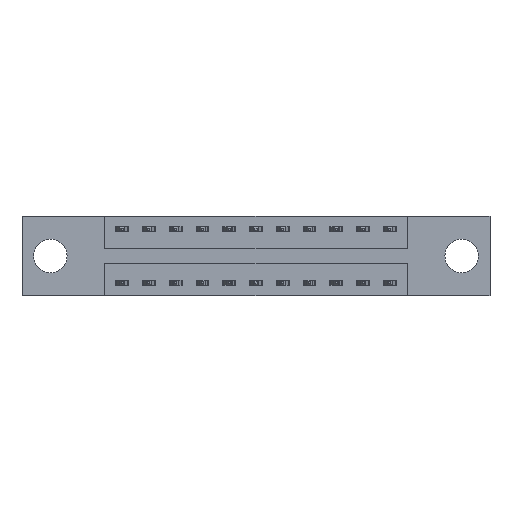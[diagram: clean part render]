
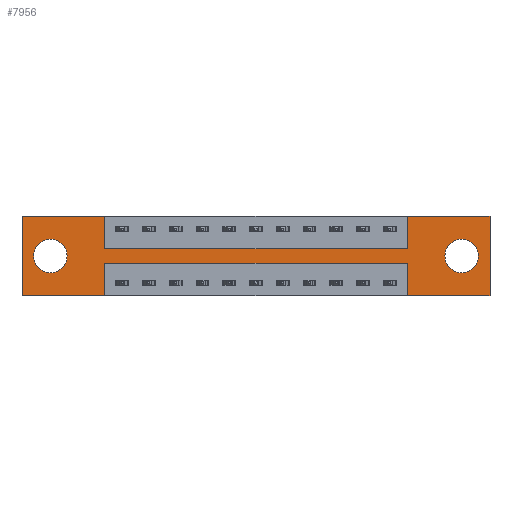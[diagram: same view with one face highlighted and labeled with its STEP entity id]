
A CAD part, front view. The second image highlights one B-rep face of the part: STEP entity #7956.
In plain terms, the highlighted planar face has unit normal (0, -1, 0).
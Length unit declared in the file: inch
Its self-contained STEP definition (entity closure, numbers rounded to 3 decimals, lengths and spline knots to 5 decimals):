
#3 = VERTEX_POINT ( 'NONE', #10753 ) ;
#63 = CARTESIAN_POINT ( 'NONE',  ( 0., 0., 0. ) ) ;
#171 = VECTOR ( 'NONE', #5956, 39.37008 ) ;
#197 = AXIS2_PLACEMENT_3D ( 'NONE', #10692, #4451, #8033 ) ;
#284 = CARTESIAN_POINT ( 'NONE',  ( 0.3875, 0., -0.22 ) ) ;
#301 = VERTEX_POINT ( 'NONE', #1676 ) ;
#316 = LINE ( 'NONE', #10496, #5406 ) ;
#406 = DIRECTION ( 'NONE',  ( 0., 1., 0. ) ) ;
#453 = ORIENTED_EDGE ( 'NONE', *, *, #6720, .F. ) ;
#528 = LINE ( 'NONE', #2189, #7311 ) ;
#599 = EDGE_CURVE ( 'NONE', #2090, #2115, #6067, .T. ) ;
#660 = PLANE ( 'NONE',  #197 ) ;
#682 = EDGE_CURVE ( 'NONE', #7720, #2903, #2788, .T. ) ;
#719 = EDGE_CURVE ( 'NONE', #2115, #2090, #3470, .T. ) ;
#831 = ORIENTED_EDGE ( 'NONE', *, *, #599, .T. ) ;
#849 = DIRECTION ( 'NONE',  ( 1., 0., 0. ) ) ;
#893 = DIRECTION ( 'NONE',  ( 0., 0., 1. ) ) ;
#897 = CARTESIAN_POINT ( 'NONE',  ( 0., 0., 0. ) ) ;
#911 = DIRECTION ( 'NONE',  ( 0., 0., 1. ) ) ;
#1139 = VECTOR ( 'NONE', #849, 39.37008 ) ;
#1198 = EDGE_CURVE ( 'NONE', #301, #8173, #5042, .T. ) ;
#1199 = DIRECTION ( 'NONE',  ( 0., 0., -1. ) ) ;
#1268 = DIRECTION ( 'NONE',  ( 0., 0., 1. ) ) ;
#1390 = DIRECTION ( 'NONE',  ( 0., 0., 1. ) ) ;
#1467 = VERTEX_POINT ( 'NONE', #3126 ) ;
#1552 = EDGE_CURVE ( 'NONE', #8173, #11756, #1583, .T. ) ;
#1583 = LINE ( 'NONE', #8945, #7128 ) ;
#1618 = ORIENTED_EDGE ( 'NONE', *, *, #719, .T. ) ;
#1676 = CARTESIAN_POINT ( 'NONE',  ( 1.7975, 0., -0.22 ) ) ;
#1816 = CARTESIAN_POINT ( 'NONE',  ( 2.0525, 0., -0.185 ) ) ;
#1943 = EDGE_CURVE ( 'NONE', #8447, #10430, #528, .T. ) ;
#2009 = EDGE_LOOP ( 'NONE', ( #1618, #831 ) ) ;
#2090 = VERTEX_POINT ( 'NONE', #11554 ) ;
#2115 = VERTEX_POINT ( 'NONE', #11005 ) ;
#2189 = CARTESIAN_POINT ( 'NONE',  ( 1.7975, 0., 0. ) ) ;
#2198 = ORIENTED_EDGE ( 'NONE', *, *, #1943, .F. ) ;
#2272 = AXIS2_PLACEMENT_3D ( 'NONE', #1816, #10988, #4686 ) ;
#2542 = VECTOR ( 'NONE', #7176, 39.37008 ) ;
#2788 = CIRCLE ( 'NONE', #10958, 0.078 ) ;
#2804 = CARTESIAN_POINT ( 'NONE',  ( 0., 0., -0.37 ) ) ;
#2903 = VERTEX_POINT ( 'NONE', #10499 ) ;
#2908 = VERTEX_POINT ( 'NONE', #7887 ) ;
#2961 = VECTOR ( 'NONE', #8928, 39.37008 ) ;
#3126 = CARTESIAN_POINT ( 'NONE',  ( 1.7975, 0., -0.37 ) ) ;
#3278 = ORIENTED_EDGE ( 'NONE', *, *, #5797, .T. ) ;
#3384 = LINE ( 'NONE', #7021, #11102 ) ;
#3470 = CIRCLE ( 'NONE', #2272, 0.078 ) ;
#3542 = LINE ( 'NONE', #4397, #2542 ) ;
#3602 = LINE ( 'NONE', #897, #11501 ) ;
#3729 = LINE ( 'NONE', #2804, #4308 ) ;
#3768 = VECTOR ( 'NONE', #911, 39.37008 ) ;
#3975 = AXIS2_PLACEMENT_3D ( 'NONE', #11304, #406, #1199 ) ;
#4032 = DIRECTION ( 'NONE',  ( -1., 0., 0. ) ) ;
#4108 = ORIENTED_EDGE ( 'NONE', *, *, #1198, .F. ) ;
#4280 = VERTEX_POINT ( 'NONE', #6567 ) ;
#4308 = VECTOR ( 'NONE', #4515, 39.37008 ) ;
#4397 = CARTESIAN_POINT ( 'NONE',  ( 0.3875, 0., -0.15 ) ) ;
#4451 = DIRECTION ( 'NONE',  ( 0., -1., 0. ) ) ;
#4515 = DIRECTION ( 'NONE',  ( -1., 0., 0. ) ) ;
#4624 = ORIENTED_EDGE ( 'NONE', *, *, #4919, .F. ) ;
#4686 = DIRECTION ( 'NONE',  ( 0., 0., -1. ) ) ;
#4919 = EDGE_CURVE ( 'NONE', #11756, #6118, #3729, .T. ) ;
#4962 = ORIENTED_EDGE ( 'NONE', *, *, #682, .T. ) ;
#5030 = AXIS2_PLACEMENT_3D ( 'NONE', #5996, #9581, #1390 ) ;
#5042 = LINE ( 'NONE', #284, #7092 ) ;
#5107 = EDGE_CURVE ( 'NONE', #2908, #1467, #316, .T. ) ;
#5137 = VERTEX_POINT ( 'NONE', #5603 ) ;
#5223 = CIRCLE ( 'NONE', #5030, 0.078 ) ;
#5257 = CARTESIAN_POINT ( 'NONE',  ( 0.3875, 0., -0.15 ) ) ;
#5369 = CARTESIAN_POINT ( 'NONE',  ( 0.1325, 0., -0.107 ) ) ;
#5406 = VECTOR ( 'NONE', #5784, 39.37008 ) ;
#5572 = DIRECTION ( 'NONE',  ( 0., 1., 0. ) ) ;
#5603 = CARTESIAN_POINT ( 'NONE',  ( 0., 0., 0. ) ) ;
#5784 = DIRECTION ( 'NONE',  ( -1., 0., 0. ) ) ;
#5797 = EDGE_CURVE ( 'NONE', #2903, #7720, #5223, .T. ) ;
#5956 = DIRECTION ( 'NONE',  ( 0., 0., -1. ) ) ;
#5996 = CARTESIAN_POINT ( 'NONE',  ( 0.1325, 0., -0.185 ) ) ;
#6010 = CARTESIAN_POINT ( 'NONE',  ( 0.3875, 0., -0.37 ) ) ;
#6067 = CIRCLE ( 'NONE', #3975, 0.078 ) ;
#6118 = VERTEX_POINT ( 'NONE', #7252 ) ;
#6434 = ORIENTED_EDGE ( 'NONE', *, *, #8017, .F. ) ;
#6445 = ORIENTED_EDGE ( 'NONE', *, *, #1552, .F. ) ;
#6567 = CARTESIAN_POINT ( 'NONE',  ( 0.3875, 0., 0. ) ) ;
#6720 = EDGE_CURVE ( 'NONE', #4280, #11645, #8645, .T. ) ;
#6988 = CARTESIAN_POINT ( 'NONE',  ( 0.1325, 0., -0.185 ) ) ;
#7021 = CARTESIAN_POINT ( 'NONE',  ( 1.7975, 0., -0.37 ) ) ;
#7092 = VECTOR ( 'NONE', #4032, 39.37008 ) ;
#7108 = DIRECTION ( 'NONE',  ( 0., 0., -1. ) ) ;
#7128 = VECTOR ( 'NONE', #7108, 39.37008 ) ;
#7176 = DIRECTION ( 'NONE',  ( 1., 0., 0. ) ) ;
#7252 = CARTESIAN_POINT ( 'NONE',  ( 0., 0., -0.37 ) ) ;
#7311 = VECTOR ( 'NONE', #1268, 39.37008 ) ;
#7344 = LINE ( 'NONE', #63, #1139 ) ;
#7414 = CARTESIAN_POINT ( 'NONE',  ( 1.7975, 0., 0. ) ) ;
#7705 = ORIENTED_EDGE ( 'NONE', *, *, #11022, .F. ) ;
#7720 = VERTEX_POINT ( 'NONE', #5369 ) ;
#7844 = CARTESIAN_POINT ( 'NONE',  ( 1.7975, 0., -0.15 ) ) ;
#7887 = CARTESIAN_POINT ( 'NONE',  ( 2.185, 0., -0.37 ) ) ;
#7956 = ADVANCED_FACE ( 'NONE', ( #11494, #9810, #8873 ), #660, .T. ) ;
#8017 = EDGE_CURVE ( 'NONE', #5137, #4280, #7344, .T. ) ;
#8030 = ORIENTED_EDGE ( 'NONE', *, *, #10691, .F. ) ;
#8033 = DIRECTION ( 'NONE',  ( 0., 0., -1. ) ) ;
#8098 = ORIENTED_EDGE ( 'NONE', *, *, #9677, .F. ) ;
#8167 = CARTESIAN_POINT ( 'NONE',  ( 0., 0., 0. ) ) ;
#8173 = VERTEX_POINT ( 'NONE', #9857 ) ;
#8220 = ORIENTED_EDGE ( 'NONE', *, *, #5107, .F. ) ;
#8447 = VERTEX_POINT ( 'NONE', #7844 ) ;
#8493 = ORIENTED_EDGE ( 'NONE', *, *, #10370, .F. ) ;
#8516 = EDGE_LOOP ( 'NONE', ( #4962, #3278 ) ) ;
#8645 = LINE ( 'NONE', #11258, #171 ) ;
#8686 = LINE ( 'NONE', #10756, #2961 ) ;
#8844 = DIRECTION ( 'NONE',  ( 0., 0., 1. ) ) ;
#8873 = FACE_OUTER_BOUND ( 'NONE', #9773, .T. ) ;
#8928 = DIRECTION ( 'NONE',  ( 0., 0., -1. ) ) ;
#8945 = CARTESIAN_POINT ( 'NONE',  ( 0.3875, 0., -0.37 ) ) ;
#9067 = DIRECTION ( 'NONE',  ( 1., 0., 0. ) ) ;
#9078 = LINE ( 'NONE', #8167, #3768 ) ;
#9581 = DIRECTION ( 'NONE',  ( 0., 1., 0. ) ) ;
#9677 = EDGE_CURVE ( 'NONE', #11645, #8447, #3542, .T. ) ;
#9773 = EDGE_LOOP ( 'NONE', ( #6445, #4108, #8493, #8220, #8030, #7705, #2198, #8098, #453, #6434, #11487, #4624 ) ) ;
#9810 = FACE_BOUND ( 'NONE', #8516, .T. ) ;
#9857 = CARTESIAN_POINT ( 'NONE',  ( 0.3875, 0., -0.22 ) ) ;
#10370 = EDGE_CURVE ( 'NONE', #1467, #301, #3384, .T. ) ;
#10430 = VERTEX_POINT ( 'NONE', #7414 ) ;
#10496 = CARTESIAN_POINT ( 'NONE',  ( 0., 0., -0.37 ) ) ;
#10499 = CARTESIAN_POINT ( 'NONE',  ( 0.1325, 0., -0.263 ) ) ;
#10691 = EDGE_CURVE ( 'NONE', #3, #2908, #8686, .T. ) ;
#10692 = CARTESIAN_POINT ( 'NONE',  ( 0., 0., -0.37 ) ) ;
#10753 = CARTESIAN_POINT ( 'NONE',  ( 2.185, 0., 0. ) ) ;
#10756 = CARTESIAN_POINT ( 'NONE',  ( 2.185, 0., 0. ) ) ;
#10958 = AXIS2_PLACEMENT_3D ( 'NONE', #6988, #5572, #893 ) ;
#10988 = DIRECTION ( 'NONE',  ( 0., 1., 0. ) ) ;
#11005 = CARTESIAN_POINT ( 'NONE',  ( 2.0525, 0., -0.107 ) ) ;
#11022 = EDGE_CURVE ( 'NONE', #10430, #3, #3602, .T. ) ;
#11102 = VECTOR ( 'NONE', #8844, 39.37008 ) ;
#11258 = CARTESIAN_POINT ( 'NONE',  ( 0.3875, 0., 0. ) ) ;
#11304 = CARTESIAN_POINT ( 'NONE',  ( 2.0525, 0., -0.185 ) ) ;
#11487 = ORIENTED_EDGE ( 'NONE', *, *, #11772, .F. ) ;
#11494 = FACE_BOUND ( 'NONE', #2009, .T. ) ;
#11501 = VECTOR ( 'NONE', #9067, 39.37008 ) ;
#11554 = CARTESIAN_POINT ( 'NONE',  ( 2.0525, 0., -0.263 ) ) ;
#11645 = VERTEX_POINT ( 'NONE', #5257 ) ;
#11756 = VERTEX_POINT ( 'NONE', #6010 ) ;
#11772 = EDGE_CURVE ( 'NONE', #6118, #5137, #9078, .T. ) ;
